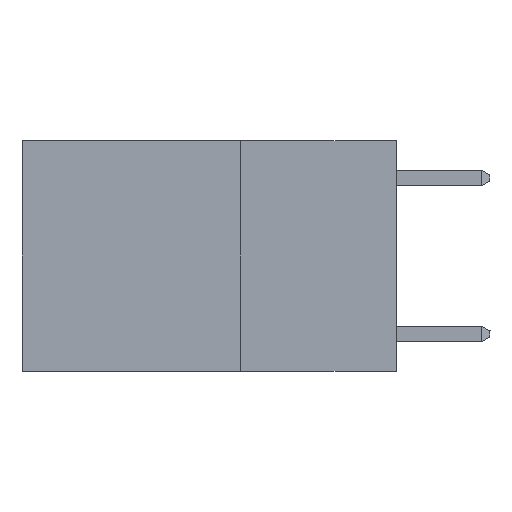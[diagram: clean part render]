
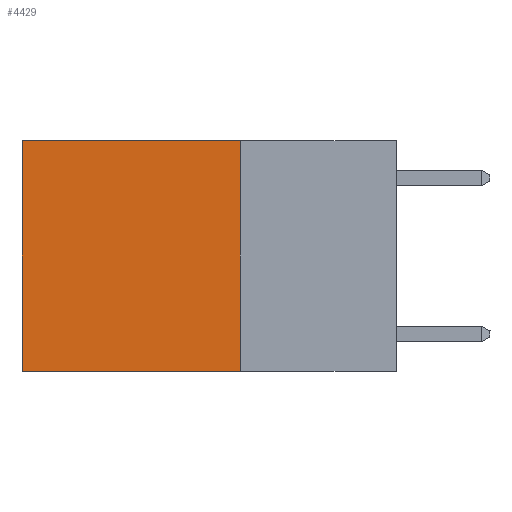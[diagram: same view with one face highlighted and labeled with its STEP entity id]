
A CAD part, left-side view. The second image highlights one B-rep face of the part: STEP entity #4429.
In plain terms, the highlighted planar face has unit normal (-1, 0, 0).
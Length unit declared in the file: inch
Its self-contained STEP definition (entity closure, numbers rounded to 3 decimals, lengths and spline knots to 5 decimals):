
#409 = EDGE_CURVE ( 'NONE', #8597, #10272, #4001, .T. ) ;
#487 = CARTESIAN_POINT ( 'NONE',  ( 0.2625, 0.25, 0. ) ) ;
#632 = CARTESIAN_POINT ( 'NONE',  ( 0.2625, 0.6, -0.37 ) ) ;
#1440 = DIRECTION ( 'NONE',  ( 0., 0., -1. ) ) ;
#1637 = VECTOR ( 'NONE', #2156, 39.37008 ) ;
#1924 = CARTESIAN_POINT ( 'NONE',  ( 0.2625, 0.25, 0. ) ) ;
#1926 = VERTEX_POINT ( 'NONE', #632 ) ;
#2156 = DIRECTION ( 'NONE',  ( 0., 0., -1. ) ) ;
#2238 = VECTOR ( 'NONE', #4750, 39.37008 ) ;
#2552 = CARTESIAN_POINT ( 'NONE',  ( 0.2625, 0.25, -0.37 ) ) ;
#3114 = DIRECTION ( 'NONE',  ( 0., 0., -1. ) ) ;
#3152 = CARTESIAN_POINT ( 'NONE',  ( 0.2625, 0.6, 0. ) ) ;
#3819 = FACE_OUTER_BOUND ( 'NONE', #7207, .T. ) ;
#4001 = LINE ( 'NONE', #10126, #1637 ) ;
#4218 = CARTESIAN_POINT ( 'NONE',  ( 0.2625, 0.6, 0. ) ) ;
#4429 = ADVANCED_FACE ( 'NONE', ( #3819 ), #5873, .F. ) ;
#4577 = LINE ( 'NONE', #1924, #2238 ) ;
#4750 = DIRECTION ( 'NONE',  ( 0., 1., 0. ) ) ;
#4950 = CARTESIAN_POINT ( 'NONE',  ( 0.2625, 0.25, 0. ) ) ;
#5873 = PLANE ( 'NONE',  #9911 ) ;
#6441 = ORIENTED_EDGE ( 'NONE', *, *, #8969, .T. ) ;
#6528 = ORIENTED_EDGE ( 'NONE', *, *, #9816, .F. ) ;
#6552 = ORIENTED_EDGE ( 'NONE', *, *, #409, .F. ) ;
#6586 = ORIENTED_EDGE ( 'NONE', *, *, #7158, .T. ) ;
#6774 = DIRECTION ( 'NONE',  ( 1., 0., 0. ) ) ;
#7060 = VERTEX_POINT ( 'NONE', #4218 ) ;
#7158 = EDGE_CURVE ( 'NONE', #8597, #7060, #4577, .T. ) ;
#7207 = EDGE_LOOP ( 'NONE', ( #6441, #6528, #6552, #6586 ) ) ;
#7328 = VECTOR ( 'NONE', #10334, 39.37008 ) ;
#8001 = CARTESIAN_POINT ( 'NONE',  ( 0.2625, 0.25, -0.37 ) ) ;
#8597 = VERTEX_POINT ( 'NONE', #4950 ) ;
#8969 = EDGE_CURVE ( 'NONE', #7060, #1926, #9042, .T. ) ;
#9042 = LINE ( 'NONE', #3152, #10472 ) ;
#9574 = LINE ( 'NONE', #2552, #7328 ) ;
#9816 = EDGE_CURVE ( 'NONE', #10272, #1926, #9574, .T. ) ;
#9911 = AXIS2_PLACEMENT_3D ( 'NONE', #487, #6774, #1440 ) ;
#10126 = CARTESIAN_POINT ( 'NONE',  ( 0.2625, 0.25, 0. ) ) ;
#10272 = VERTEX_POINT ( 'NONE', #8001 ) ;
#10334 = DIRECTION ( 'NONE',  ( 0., 1., 0. ) ) ;
#10472 = VECTOR ( 'NONE', #3114, 39.37008 ) ;
